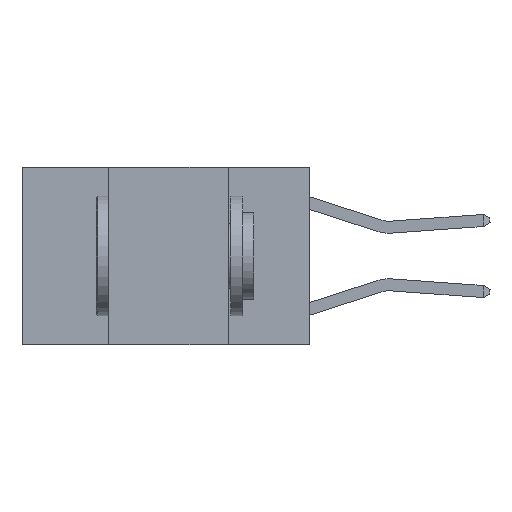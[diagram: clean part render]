
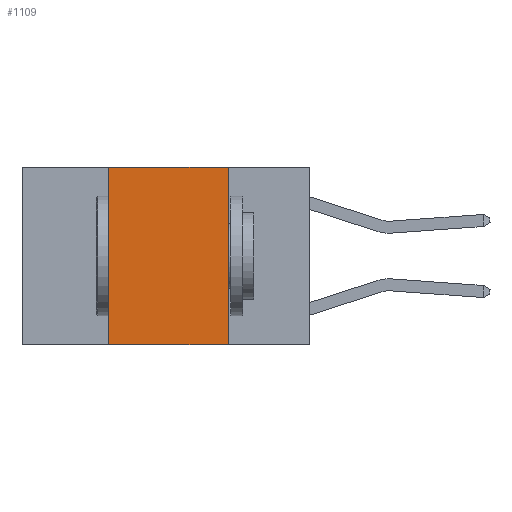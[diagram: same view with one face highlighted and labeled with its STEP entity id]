
A CAD part, left-side view. The second image highlights one B-rep face of the part: STEP entity #1109.
In plain terms, the highlighted planar face has unit normal (-1, 0, 0).
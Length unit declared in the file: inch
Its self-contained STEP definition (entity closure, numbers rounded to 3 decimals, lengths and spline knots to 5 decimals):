
#92 = VERTEX_POINT ( 'NONE', #8232 ) ;
#185 = EDGE_CURVE ( 'NONE', #8931, #12056, #7573, .T. ) ;
#278 = EDGE_CURVE ( 'NONE', #1147, #92, #3546, .T. ) ;
#500 = PLANE ( 'NONE',  #11230 ) ;
#1109 = ADVANCED_FACE ( 'NONE', ( #10959 ), #500, .F. ) ;
#1147 = VERTEX_POINT ( 'NONE', #4886 ) ;
#2680 = DIRECTION ( 'NONE',  ( 0., -1., 0. ) ) ;
#3546 = LINE ( 'NONE', #10988, #9541 ) ;
#3675 = LINE ( 'NONE', #6484, #9144 ) ;
#4426 = VECTOR ( 'NONE', #11444, 39.37008 ) ;
#4622 = ORIENTED_EDGE ( 'NONE', *, *, #7535, .T. ) ;
#4836 = EDGE_LOOP ( 'NONE', ( #7193, #8650, #8394, #4622 ) ) ;
#4886 = CARTESIAN_POINT ( 'NONE',  ( 0., 0.17, 0. ) ) ;
#6249 = CARTESIAN_POINT ( 'NONE',  ( 0., 0.6, 0. ) ) ;
#6365 = VECTOR ( 'NONE', #8329, 39.37008 ) ;
#6484 = CARTESIAN_POINT ( 'NONE',  ( 0., 0.6, 0. ) ) ;
#7137 = EDGE_CURVE ( 'NONE', #12056, #1147, #3675, .T. ) ;
#7193 = ORIENTED_EDGE ( 'NONE', *, *, #278, .F. ) ;
#7258 = CARTESIAN_POINT ( 'NONE',  ( 0., 0.42, 0. ) ) ;
#7518 = CARTESIAN_POINT ( 'NONE',  ( 0., 0.6, -0.37 ) ) ;
#7521 = CARTESIAN_POINT ( 'NONE',  ( 0., 0.42, -0.37 ) ) ;
#7535 = EDGE_CURVE ( 'NONE', #8931, #92, #8404, .T. ) ;
#7573 = LINE ( 'NONE', #9551, #4426 ) ;
#8232 = CARTESIAN_POINT ( 'NONE',  ( 0., 0.17, -0.37 ) ) ;
#8329 = DIRECTION ( 'NONE',  ( 0., -1., 0. ) ) ;
#8394 = ORIENTED_EDGE ( 'NONE', *, *, #185, .F. ) ;
#8404 = LINE ( 'NONE', #7518, #6365 ) ;
#8650 = ORIENTED_EDGE ( 'NONE', *, *, #7137, .F. ) ;
#8931 = VERTEX_POINT ( 'NONE', #7521 ) ;
#9144 = VECTOR ( 'NONE', #2680, 39.37008 ) ;
#9541 = VECTOR ( 'NONE', #10863, 39.37008 ) ;
#9551 = CARTESIAN_POINT ( 'NONE',  ( 0., 0.42, 0. ) ) ;
#9793 = DIRECTION ( 'NONE',  ( 1., 0., 0. ) ) ;
#10863 = DIRECTION ( 'NONE',  ( 0., 0., -1. ) ) ;
#10959 = FACE_OUTER_BOUND ( 'NONE', #4836, .T. ) ;
#10988 = CARTESIAN_POINT ( 'NONE',  ( 0., 0.17, 0. ) ) ;
#11230 = AXIS2_PLACEMENT_3D ( 'NONE', #6249, #9793, #11701 ) ;
#11444 = DIRECTION ( 'NONE',  ( 0., 0., 1. ) ) ;
#11701 = DIRECTION ( 'NONE',  ( 0., 0., -1. ) ) ;
#12056 = VERTEX_POINT ( 'NONE', #7258 ) ;
